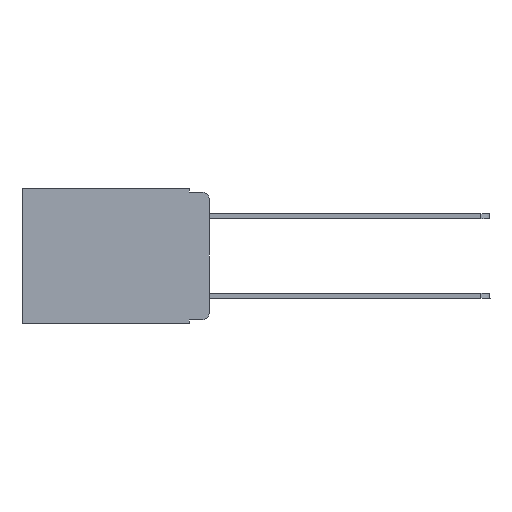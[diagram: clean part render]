
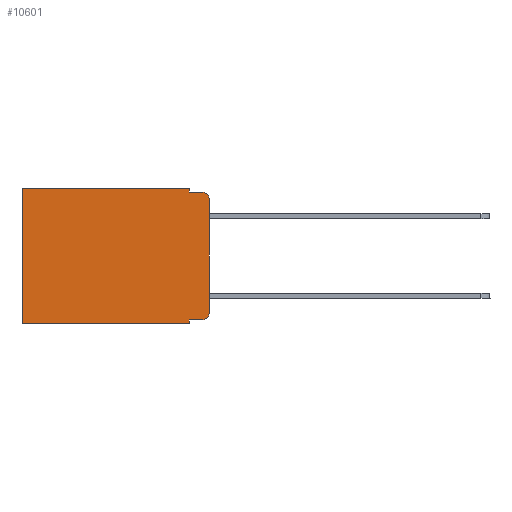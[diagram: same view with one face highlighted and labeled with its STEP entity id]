
A CAD part, left-side view. The second image highlights one B-rep face of the part: STEP entity #10601.
In plain terms, the highlighted planar face has unit normal (-1, 0, 0).
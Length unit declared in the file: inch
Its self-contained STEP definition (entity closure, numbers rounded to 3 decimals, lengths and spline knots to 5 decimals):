
#285 = ORIENTED_EDGE ( 'NONE', *, *, #7548, .F. ) ;
#306 = LINE ( 'NONE', #2530, #5419 ) ;
#357 = ORIENTED_EDGE ( 'NONE', *, *, #7247, .T. ) ;
#575 = ORIENTED_EDGE ( 'NONE', *, *, #9448, .T. ) ;
#743 = CIRCLE ( 'NONE', #9813, 0.02 ) ;
#966 = CARTESIAN_POINT ( 'NONE',  ( 0.298, 0.051, -0.333 ) ) ;
#1061 = VECTOR ( 'NONE', #5493, 39.37008 ) ;
#1138 = DIRECTION ( 'NONE',  ( 0., 0., -1. ) ) ;
#1223 = LINE ( 'NONE', #6684, #4578 ) ;
#1513 = LINE ( 'NONE', #4460, #10992 ) ;
#1517 = DIRECTION ( 'NONE',  ( 0., 0., -1. ) ) ;
#1733 = DIRECTION ( 'NONE',  ( 0., 0., -1. ) ) ;
#1847 = CARTESIAN_POINT ( 'NONE',  ( 0.298, 0.051, -0.01 ) ) ;
#1869 = EDGE_CURVE ( 'NONE', #10805, #2091, #6931, .T. ) ;
#2091 = VERTEX_POINT ( 'NONE', #8186 ) ;
#2177 = CARTESIAN_POINT ( 'NONE',  ( 0.298, 0., 0. ) ) ;
#2196 = VERTEX_POINT ( 'NONE', #4711 ) ;
#2453 = DIRECTION ( 'NONE',  ( -1., 0., 0. ) ) ;
#2530 = CARTESIAN_POINT ( 'NONE',  ( 0.298, 0., 0. ) ) ;
#2689 = EDGE_CURVE ( 'NONE', #11938, #2196, #3026, .T. ) ;
#2716 = VECTOR ( 'NONE', #6794, 39.37008 ) ;
#2761 = EDGE_CURVE ( 'NONE', #3573, #6443, #8355, .T. ) ;
#3026 = LINE ( 'NONE', #12949, #2716 ) ;
#3151 = CARTESIAN_POINT ( 'NONE',  ( 0.298, 0.473, 0. ) ) ;
#3186 = EDGE_CURVE ( 'NONE', #9039, #10050, #306, .T. ) ;
#3243 = CARTESIAN_POINT ( 'NONE',  ( 0.298, 0., -0.03 ) ) ;
#3385 = VECTOR ( 'NONE', #5671, 39.37008 ) ;
#3496 = CARTESIAN_POINT ( 'NONE',  ( 0.298, 0.051, 0. ) ) ;
#3573 = VERTEX_POINT ( 'NONE', #11866 ) ;
#3658 = DIRECTION ( 'NONE',  ( 0., 0., -1. ) ) ;
#3699 = ORIENTED_EDGE ( 'NONE', *, *, #5223, .F. ) ;
#3915 = ORIENTED_EDGE ( 'NONE', *, *, #3186, .T. ) ;
#4127 = DIRECTION ( 'NONE',  ( 1., 0., 0. ) ) ;
#4433 = CARTESIAN_POINT ( 'NONE',  ( 0.298, 0.051, 0. ) ) ;
#4460 = CARTESIAN_POINT ( 'NONE',  ( 0.298, 0.473, 0. ) ) ;
#4571 = EDGE_CURVE ( 'NONE', #10034, #9241, #1223, .T. ) ;
#4578 = VECTOR ( 'NONE', #3658, 39.37008 ) ;
#4711 = CARTESIAN_POINT ( 'NONE',  ( 0.298, 0.473, -0.343 ) ) ;
#5223 = EDGE_CURVE ( 'NONE', #3573, #11938, #6376, .T. ) ;
#5297 = PLANE ( 'NONE',  #8299 ) ;
#5419 = VECTOR ( 'NONE', #7663, 39.37008 ) ;
#5493 = DIRECTION ( 'NONE',  ( 0., 0., -1. ) ) ;
#5671 = DIRECTION ( 'NONE',  ( 0., -1., 0. ) ) ;
#6171 = VECTOR ( 'NONE', #12642, 39.37008 ) ;
#6376 = LINE ( 'NONE', #3496, #1061 ) ;
#6443 = VERTEX_POINT ( 'NONE', #11038 ) ;
#6684 = CARTESIAN_POINT ( 'NONE',  ( 0.298, 0., 0. ) ) ;
#6685 = CARTESIAN_POINT ( 'NONE',  ( 0.298, 0.02, -0.313 ) ) ;
#6734 = CARTESIAN_POINT ( 'NONE',  ( 0.298, 0.051, -0.01 ) ) ;
#6794 = DIRECTION ( 'NONE',  ( 0., 1., 0. ) ) ;
#6819 = DIRECTION ( 'NONE',  ( -1., 0., 0. ) ) ;
#6931 = LINE ( 'NONE', #6734, #3385 ) ;
#7040 = AXIS2_PLACEMENT_3D ( 'NONE', #7811, #6819, #1733 ) ;
#7247 = EDGE_CURVE ( 'NONE', #10034, #2091, #10195, .T. ) ;
#7548 = EDGE_CURVE ( 'NONE', #9039, #10805, #10359, .T. ) ;
#7663 = DIRECTION ( 'NONE',  ( 0., 1., 0. ) ) ;
#7811 = CARTESIAN_POINT ( 'NONE',  ( 0.298, 0.02, -0.03 ) ) ;
#7913 = EDGE_CURVE ( 'NONE', #10050, #2196, #1513, .T. ) ;
#8186 = CARTESIAN_POINT ( 'NONE',  ( 0.298, 0.02, -0.01 ) ) ;
#8288 = ORIENTED_EDGE ( 'NONE', *, *, #7913, .T. ) ;
#8299 = AXIS2_PLACEMENT_3D ( 'NONE', #2177, #4127, #1138 ) ;
#8355 = LINE ( 'NONE', #966, #10929 ) ;
#8514 = ORIENTED_EDGE ( 'NONE', *, *, #4571, .F. ) ;
#9039 = VERTEX_POINT ( 'NONE', #11944 ) ;
#9241 = VERTEX_POINT ( 'NONE', #12553 ) ;
#9260 = ORIENTED_EDGE ( 'NONE', *, *, #2689, .F. ) ;
#9448 = EDGE_CURVE ( 'NONE', #6443, #9241, #743, .T. ) ;
#9760 = DIRECTION ( 'NONE',  ( 0., 0., -1. ) ) ;
#9813 = AXIS2_PLACEMENT_3D ( 'NONE', #6685, #2453, #1517 ) ;
#10034 = VERTEX_POINT ( 'NONE', #3243 ) ;
#10050 = VERTEX_POINT ( 'NONE', #3151 ) ;
#10128 = CARTESIAN_POINT ( 'NONE',  ( 0.298, 0.051, -0.343 ) ) ;
#10195 = CIRCLE ( 'NONE', #7040, 0.02 ) ;
#10359 = LINE ( 'NONE', #4433, #6171 ) ;
#10488 = FACE_OUTER_BOUND ( 'NONE', #11500, .T. ) ;
#10601 = ADVANCED_FACE ( 'NONE', ( #10488 ), #5297, .F. ) ;
#10787 = ORIENTED_EDGE ( 'NONE', *, *, #1869, .F. ) ;
#10805 = VERTEX_POINT ( 'NONE', #1847 ) ;
#10929 = VECTOR ( 'NONE', #11188, 39.37008 ) ;
#10992 = VECTOR ( 'NONE', #9760, 39.37008 ) ;
#11038 = CARTESIAN_POINT ( 'NONE',  ( 0.298, 0.02, -0.333 ) ) ;
#11188 = DIRECTION ( 'NONE',  ( 0., -1., 0. ) ) ;
#11500 = EDGE_LOOP ( 'NONE', ( #8514, #357, #10787, #285, #3915, #8288, #9260, #3699, #12158, #575 ) ) ;
#11866 = CARTESIAN_POINT ( 'NONE',  ( 0.298, 0.051, -0.333 ) ) ;
#11938 = VERTEX_POINT ( 'NONE', #10128 ) ;
#11944 = CARTESIAN_POINT ( 'NONE',  ( 0.298, 0.051, 0. ) ) ;
#12158 = ORIENTED_EDGE ( 'NONE', *, *, #2761, .T. ) ;
#12553 = CARTESIAN_POINT ( 'NONE',  ( 0.298, 0., -0.313 ) ) ;
#12642 = DIRECTION ( 'NONE',  ( 0., 0., -1. ) ) ;
#12949 = CARTESIAN_POINT ( 'NONE',  ( 0.298, 0., -0.343 ) ) ;
